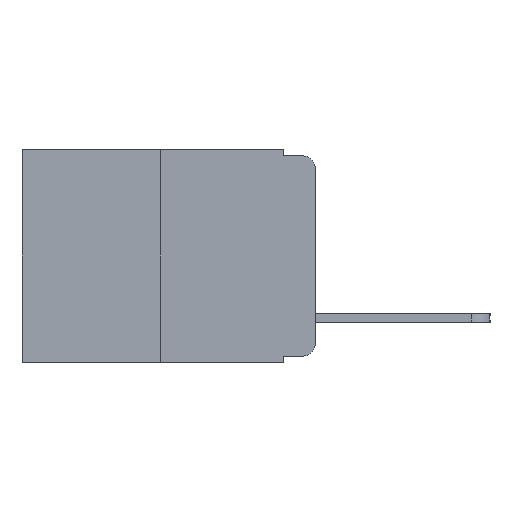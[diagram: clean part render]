
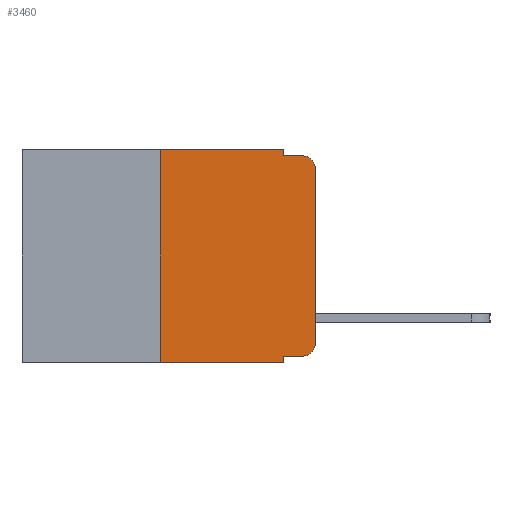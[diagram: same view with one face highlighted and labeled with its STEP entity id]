
A CAD part, left-side view. The second image highlights one B-rep face of the part: STEP entity #3460.
In plain terms, the highlighted planar face has unit normal (-1, 0, 0).
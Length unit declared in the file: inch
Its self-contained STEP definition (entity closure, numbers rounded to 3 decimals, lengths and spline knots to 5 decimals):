
#82 = LINE ( 'NONE', #11031, #7221 ) ;
#288 = CIRCLE ( 'NONE', #9470, 0.02 ) ;
#360 = CARTESIAN_POINT ( 'NONE',  ( 0., 0., -0.313 ) ) ;
#503 = CARTESIAN_POINT ( 'NONE',  ( 0., 0.051, 0. ) ) ;
#512 = DIRECTION ( 'NONE',  ( 0., 0., -1. ) ) ;
#629 = EDGE_CURVE ( 'NONE', #2336, #2066, #5218, .T. ) ;
#887 = CARTESIAN_POINT ( 'NONE',  ( 0., 0.051, -0.333 ) ) ;
#922 = EDGE_CURVE ( 'NONE', #3835, #8583, #82, .T. ) ;
#1197 = LINE ( 'NONE', #2366, #10424 ) ;
#1748 = CARTESIAN_POINT ( 'NONE',  ( 0., 0., 0. ) ) ;
#1776 = EDGE_CURVE ( 'NONE', #8583, #2336, #1197, .T. ) ;
#1824 = LINE ( 'NONE', #1748, #6481 ) ;
#2066 = VERTEX_POINT ( 'NONE', #6217 ) ;
#2097 = CARTESIAN_POINT ( 'NONE',  ( 0., 0.051, -0.01 ) ) ;
#2302 = VERTEX_POINT ( 'NONE', #2308 ) ;
#2308 = CARTESIAN_POINT ( 'NONE',  ( 0., 0.02, -0.333 ) ) ;
#2336 = VERTEX_POINT ( 'NONE', #2097 ) ;
#2366 = CARTESIAN_POINT ( 'NONE',  ( 0., 0.051, 0. ) ) ;
#2628 = LINE ( 'NONE', #887, #8778 ) ;
#2798 = VERTEX_POINT ( 'NONE', #8191 ) ;
#2844 = DIRECTION ( 'NONE',  ( 0., -1., 0. ) ) ;
#3223 = EDGE_LOOP ( 'NONE', ( #5365, #6331, #6465, #7367, #7499, #8223, #8348, #9209, #9447, #10054 ) ) ;
#3392 = EDGE_CURVE ( 'NONE', #2302, #9242, #288, .T. ) ;
#3460 = ADVANCED_FACE ( 'NONE', ( #7113 ), #10072, .F. ) ;
#3536 = EDGE_CURVE ( 'NONE', #6070, #3566, #3917, .T. ) ;
#3566 = VERTEX_POINT ( 'NONE', #5135 ) ;
#3835 = VERTEX_POINT ( 'NONE', #10232 ) ;
#3841 = EDGE_CURVE ( 'NONE', #5937, #2066, #5079, .T. ) ;
#3917 = LINE ( 'NONE', #4431, #8237 ) ;
#4431 = CARTESIAN_POINT ( 'NONE',  ( 0., 0.051, 0. ) ) ;
#4833 = VECTOR ( 'NONE', #10351, 39.37008 ) ;
#4845 = AXIS2_PLACEMENT_3D ( 'NONE', #10017, #8516, #11135 ) ;
#5079 = CIRCLE ( 'NONE', #7313, 0.02 ) ;
#5135 = CARTESIAN_POINT ( 'NONE',  ( 0., 0.051, -0.343 ) ) ;
#5218 = LINE ( 'NONE', #8041, #9334 ) ;
#5365 = ORIENTED_EDGE ( 'NONE', *, *, #10386, .T. ) ;
#5736 = CARTESIAN_POINT ( 'NONE',  ( 0., 0.02, -0.313 ) ) ;
#5750 = DIRECTION ( 'NONE',  ( -1., 0., 0. ) ) ;
#5847 = VECTOR ( 'NONE', #2844, 39.37008 ) ;
#5937 = VERTEX_POINT ( 'NONE', #9020 ) ;
#6070 = VERTEX_POINT ( 'NONE', #7194 ) ;
#6217 = CARTESIAN_POINT ( 'NONE',  ( 0., 0.02, -0.01 ) ) ;
#6331 = ORIENTED_EDGE ( 'NONE', *, *, #3841, .T. ) ;
#6386 = CARTESIAN_POINT ( 'NONE',  ( 0., 0.25, 0. ) ) ;
#6465 = ORIENTED_EDGE ( 'NONE', *, *, #629, .F. ) ;
#6481 = VECTOR ( 'NONE', #11113, 39.37008 ) ;
#7113 = FACE_OUTER_BOUND ( 'NONE', #3223, .T. ) ;
#7194 = CARTESIAN_POINT ( 'NONE',  ( 0., 0.051, -0.333 ) ) ;
#7221 = VECTOR ( 'NONE', #9532, 39.37008 ) ;
#7313 = AXIS2_PLACEMENT_3D ( 'NONE', #9953, #9969, #9743 ) ;
#7367 = ORIENTED_EDGE ( 'NONE', *, *, #1776, .F. ) ;
#7466 = EDGE_CURVE ( 'NONE', #6070, #2302, #2628, .T. ) ;
#7499 = ORIENTED_EDGE ( 'NONE', *, *, #922, .F. ) ;
#7799 = LINE ( 'NONE', #8927, #5847 ) ;
#8041 = CARTESIAN_POINT ( 'NONE',  ( 0., 0.051, -0.01 ) ) ;
#8136 = EDGE_CURVE ( 'NONE', #2798, #3566, #7799, .T. ) ;
#8191 = CARTESIAN_POINT ( 'NONE',  ( 0., 0.25, -0.343 ) ) ;
#8223 = ORIENTED_EDGE ( 'NONE', *, *, #9572, .F. ) ;
#8237 = VECTOR ( 'NONE', #10782, 39.37008 ) ;
#8348 = ORIENTED_EDGE ( 'NONE', *, *, #8136, .T. ) ;
#8516 = DIRECTION ( 'NONE',  ( 1., 0., 0. ) ) ;
#8583 = VERTEX_POINT ( 'NONE', #503 ) ;
#8778 = VECTOR ( 'NONE', #11255, 39.37008 ) ;
#8927 = CARTESIAN_POINT ( 'NONE',  ( 0., 0.473, -0.343 ) ) ;
#9020 = CARTESIAN_POINT ( 'NONE',  ( 0., 0., -0.03 ) ) ;
#9209 = ORIENTED_EDGE ( 'NONE', *, *, #3536, .F. ) ;
#9242 = VERTEX_POINT ( 'NONE', #360 ) ;
#9263 = DIRECTION ( 'NONE',  ( 0., -1., 0. ) ) ;
#9334 = VECTOR ( 'NONE', #9263, 39.37008 ) ;
#9447 = ORIENTED_EDGE ( 'NONE', *, *, #7466, .T. ) ;
#9470 = AXIS2_PLACEMENT_3D ( 'NONE', #5736, #5750, #11303 ) ;
#9532 = DIRECTION ( 'NONE',  ( 0., -1., 0. ) ) ;
#9572 = EDGE_CURVE ( 'NONE', #2798, #3835, #11323, .T. ) ;
#9743 = DIRECTION ( 'NONE',  ( 0., 0., -1. ) ) ;
#9953 = CARTESIAN_POINT ( 'NONE',  ( 0., 0.02, -0.03 ) ) ;
#9969 = DIRECTION ( 'NONE',  ( -1., 0., 0. ) ) ;
#10017 = CARTESIAN_POINT ( 'NONE',  ( 0., 0.473, 0. ) ) ;
#10054 = ORIENTED_EDGE ( 'NONE', *, *, #3392, .T. ) ;
#10072 = PLANE ( 'NONE',  #4845 ) ;
#10232 = CARTESIAN_POINT ( 'NONE',  ( 0., 0.25, 0. ) ) ;
#10351 = DIRECTION ( 'NONE',  ( 0., 0., 1. ) ) ;
#10386 = EDGE_CURVE ( 'NONE', #9242, #5937, #1824, .T. ) ;
#10424 = VECTOR ( 'NONE', #512, 39.37008 ) ;
#10782 = DIRECTION ( 'NONE',  ( 0., 0., -1. ) ) ;
#11031 = CARTESIAN_POINT ( 'NONE',  ( 0., 0.473, 0. ) ) ;
#11113 = DIRECTION ( 'NONE',  ( 0., 0., 1. ) ) ;
#11135 = DIRECTION ( 'NONE',  ( 0., 0., -1. ) ) ;
#11255 = DIRECTION ( 'NONE',  ( 0., -1., 0. ) ) ;
#11303 = DIRECTION ( 'NONE',  ( 0., 0., -1. ) ) ;
#11323 = LINE ( 'NONE', #6386, #4833 ) ;
